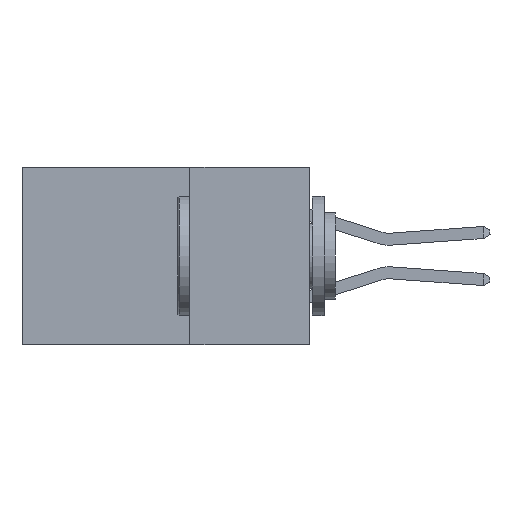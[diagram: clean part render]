
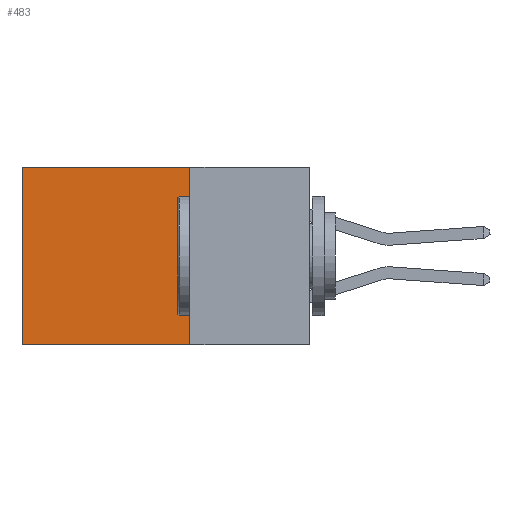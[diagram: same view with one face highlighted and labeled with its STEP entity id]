
A CAD part, left-side view. The second image highlights one B-rep face of the part: STEP entity #483.
In plain terms, the highlighted planar face has unit normal (-1, 0, 0).
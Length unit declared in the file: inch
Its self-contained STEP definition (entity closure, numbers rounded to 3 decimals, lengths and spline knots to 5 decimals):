
#412 = VECTOR ( 'NONE', #21892, 39.37008 ) ;
#483 = ADVANCED_FACE ( 'NONE', ( #5297 ), #7053, .F. ) ;
#768 = LINE ( 'NONE', #22537, #6438 ) ;
#2079 = CARTESIAN_POINT ( 'NONE',  ( 0.298, 0.6, -0.37 ) ) ;
#2289 = CARTESIAN_POINT ( 'NONE',  ( 0.298, 0.25, 0. ) ) ;
#3271 = VERTEX_POINT ( 'NONE', #13206 ) ;
#3969 = VERTEX_POINT ( 'NONE', #2079 ) ;
#4756 = ORIENTED_EDGE ( 'NONE', *, *, #10216, .T. ) ;
#5297 = FACE_OUTER_BOUND ( 'NONE', #6053, .T. ) ;
#5543 = DIRECTION ( 'NONE',  ( 0., 1., 0. ) ) ;
#5700 = DIRECTION ( 'NONE',  ( 1., 0., 0. ) ) ;
#6053 = EDGE_LOOP ( 'NONE', ( #4756, #21172, #8241, #12237 ) ) ;
#6438 = VECTOR ( 'NONE', #5543, 39.37008 ) ;
#6755 = LINE ( 'NONE', #9158, #412 ) ;
#6925 = CARTESIAN_POINT ( 'NONE',  ( 0.298, 0.25, 0. ) ) ;
#7053 = PLANE ( 'NONE',  #19878 ) ;
#8241 = ORIENTED_EDGE ( 'NONE', *, *, #15051, .F. ) ;
#9158 = CARTESIAN_POINT ( 'NONE',  ( 0.298, 0.25, 0. ) ) ;
#10167 = EDGE_CURVE ( 'NONE', #20154, #3969, #768, .T. ) ;
#10215 = CARTESIAN_POINT ( 'NONE',  ( 0.298, 0.6, 0. ) ) ;
#10216 = EDGE_CURVE ( 'NONE', #16627, #3969, #10749, .T. ) ;
#10670 = VECTOR ( 'NONE', #23472, 39.37008 ) ;
#10749 = LINE ( 'NONE', #14145, #21387 ) ;
#12237 = ORIENTED_EDGE ( 'NONE', *, *, #16820, .T. ) ;
#13206 = CARTESIAN_POINT ( 'NONE',  ( 0.298, 0.25, 0. ) ) ;
#13320 = DIRECTION ( 'NONE',  ( 0., 0., -1. ) ) ;
#14145 = CARTESIAN_POINT ( 'NONE',  ( 0.298, 0.6, 0. ) ) ;
#15051 = EDGE_CURVE ( 'NONE', #3271, #20154, #6755, .T. ) ;
#16262 = DIRECTION ( 'NONE',  ( 0., 0., -1. ) ) ;
#16627 = VERTEX_POINT ( 'NONE', #10215 ) ;
#16820 = EDGE_CURVE ( 'NONE', #3271, #16627, #21974, .T. ) ;
#19878 = AXIS2_PLACEMENT_3D ( 'NONE', #6925, #5700, #13320 ) ;
#20154 = VERTEX_POINT ( 'NONE', #23462 ) ;
#21172 = ORIENTED_EDGE ( 'NONE', *, *, #10167, .F. ) ;
#21387 = VECTOR ( 'NONE', #16262, 39.37008 ) ;
#21892 = DIRECTION ( 'NONE',  ( 0., 0., -1. ) ) ;
#21974 = LINE ( 'NONE', #2289, #10670 ) ;
#22537 = CARTESIAN_POINT ( 'NONE',  ( 0.298, 0.25, -0.37 ) ) ;
#23462 = CARTESIAN_POINT ( 'NONE',  ( 0.298, 0.25, -0.37 ) ) ;
#23472 = DIRECTION ( 'NONE',  ( 0., 1., 0. ) ) ;
